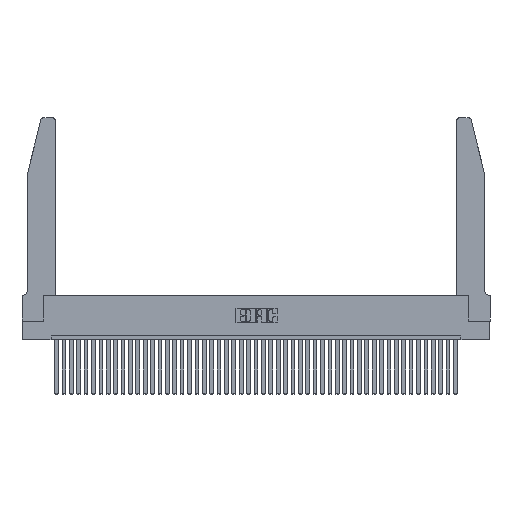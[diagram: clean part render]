
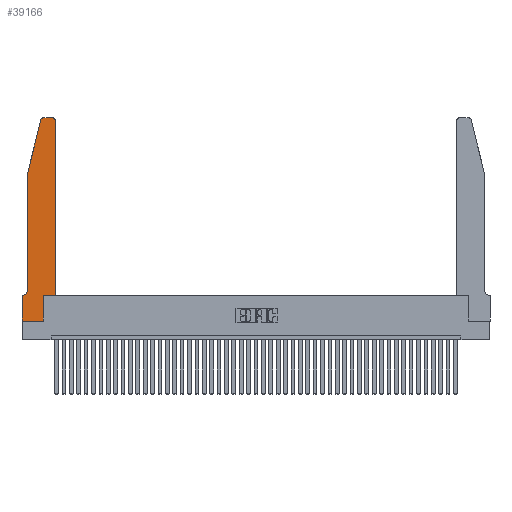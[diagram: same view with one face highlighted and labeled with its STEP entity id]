
A CAD part, top view. The second image highlights one B-rep face of the part: STEP entity #39166.
In plain terms, the highlighted planar face has unit normal (0, 0, 1).
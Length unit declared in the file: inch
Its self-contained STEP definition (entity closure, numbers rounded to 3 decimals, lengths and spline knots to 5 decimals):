
#9 = CARTESIAN_POINT ( 'NONE',  ( 0.0055, 0.42, 0.37 ) ) ;
#108 = CARTESIAN_POINT ( 'NONE',  ( 0.0755, 2., 0.37 ) ) ;
#1256 = CARTESIAN_POINT ( 'NONE',  ( 0.4205, 2.75, 0.37 ) ) ;
#1300 = DIRECTION ( 'NONE',  ( 1., 0., 0. ) ) ;
#1984 = VERTEX_POINT ( 'NONE', #10881 ) ;
#2824 = CARTESIAN_POINT ( 'NONE',  ( 0., 0.35, 0.37 ) ) ;
#2923 = LINE ( 'NONE', #6059, #33946 ) ;
#2985 = EDGE_CURVE ( 'NONE', #41878, #21738, #17395, .T. ) ;
#4377 = CARTESIAN_POINT ( 'NONE',  ( 0., 0.35, 0.37 ) ) ;
#4816 = CARTESIAN_POINT ( 'NONE',  ( 0.0755, 2., 0.37 ) ) ;
#5029 = VECTOR ( 'NONE', #18848, 39.37008 ) ;
#5049 = LINE ( 'NONE', #5074, #27039 ) ;
#5074 = CARTESIAN_POINT ( 'NONE',  ( 0.0755, 2., 0.37 ) ) ;
#5537 = VERTEX_POINT ( 'NONE', #5894 ) ;
#5815 = VERTEX_POINT ( 'NONE', #25529 ) ;
#5894 = CARTESIAN_POINT ( 'NONE',  ( 0., 0., 0.37 ) ) ;
#6059 = CARTESIAN_POINT ( 'NONE',  ( 0., 0., 0.37 ) ) ;
#7155 = VECTOR ( 'NONE', #27680, 39.37008 ) ;
#7263 = ORIENTED_EDGE ( 'NONE', *, *, #20639, .T. ) ;
#7273 = ORIENTED_EDGE ( 'NONE', *, *, #2985, .T. ) ;
#8125 = PLANE ( 'NONE',  #23287 ) ;
#8174 = DIRECTION ( 'NONE',  ( -1., 0., 0. ) ) ;
#9148 = ORIENTED_EDGE ( 'NONE', *, *, #26729, .T. ) ;
#9227 = DIRECTION ( 'NONE',  ( 0., -1., 0. ) ) ;
#9733 = EDGE_CURVE ( 'NONE', #5815, #37742, #29258, .T. ) ;
#10742 = CARTESIAN_POINT ( 'NONE',  ( 0.2605, 2.75, 0.37 ) ) ;
#10881 = CARTESIAN_POINT ( 'NONE',  ( 0.0755, 0.42, 0.37 ) ) ;
#10886 = EDGE_LOOP ( 'NONE', ( #37400, #36214, #31388, #26206, #20294, #7263, #9148, #14751, #7273, #43593, #41865, #40625 ) ) ;
#11112 = AXIS2_PLACEMENT_3D ( 'NONE', #23841, #27307, #30699 ) ;
#11327 = CARTESIAN_POINT ( 'NONE',  ( 0.4505, 0.35, 0.37 ) ) ;
#11474 = CARTESIAN_POINT ( 'NONE',  ( 0., 0., 0.37 ) ) ;
#13415 = EDGE_CURVE ( 'NONE', #23583, #5815, #24755, .T. ) ;
#13886 = LINE ( 'NONE', #4816, #30492 ) ;
#14198 = DIRECTION ( 'NONE',  ( 0., 0., -1. ) ) ;
#14213 = EDGE_CURVE ( 'NONE', #37742, #35950, #34302, .T. ) ;
#14751 = ORIENTED_EDGE ( 'NONE', *, *, #35418, .T. ) ;
#15029 = DIRECTION ( 'NONE',  ( 0., 0., 1. ) ) ;
#15263 = CARTESIAN_POINT ( 'NONE',  ( 0.4505, 0.35, 0.37 ) ) ;
#15727 = LINE ( 'NONE', #11474, #39719 ) ;
#17077 = DIRECTION ( 'NONE',  ( -1., 0., 0. ) ) ;
#17395 = LINE ( 'NONE', #36255, #5029 ) ;
#18848 = DIRECTION ( 'NONE',  ( 0., 1., 0. ) ) ;
#19045 = CIRCLE ( 'NONE', #31973, 0.07 ) ;
#19612 = DIRECTION ( 'NONE',  ( 1., 0., 0. ) ) ;
#19721 = CARTESIAN_POINT ( 'NONE',  ( 0.25487, 2.72718, 0.37 ) ) ;
#20294 = ORIENTED_EDGE ( 'NONE', *, *, #34423, .T. ) ;
#20495 = EDGE_CURVE ( 'NONE', #31347, #23967, #5049, .T. ) ;
#20639 = EDGE_CURVE ( 'NONE', #40526, #27176, #22181, .T. ) ;
#21601 = CARTESIAN_POINT ( 'NONE',  ( 0.2865, 0., 0.37 ) ) ;
#21650 = DIRECTION ( 'NONE',  ( 0., 1., 0. ) ) ;
#21738 = VERTEX_POINT ( 'NONE', #36974 ) ;
#22181 = LINE ( 'NONE', #30496, #7155 ) ;
#22701 = CARTESIAN_POINT ( 'NONE',  ( 0.0055, 0.35, 0.37 ) ) ;
#23287 = AXIS2_PLACEMENT_3D ( 'NONE', #4377, #15029, #38877 ) ;
#23583 = VERTEX_POINT ( 'NONE', #15263 ) ;
#23841 = CARTESIAN_POINT ( 'NONE',  ( 0.4205, 2.72, 0.37 ) ) ;
#23967 = VERTEX_POINT ( 'NONE', #108 ) ;
#24738 = CARTESIAN_POINT ( 'NONE',  ( 0.284, 2.75, 0.37 ) ) ;
#24755 = LINE ( 'NONE', #11327, #42322 ) ;
#24767 = VECTOR ( 'NONE', #42354, 39.37008 ) ;
#25082 = CARTESIAN_POINT ( 'NONE',  ( 0.4505, 0.35, 0.37 ) ) ;
#25529 = CARTESIAN_POINT ( 'NONE',  ( 0.4505, 2.72, 0.37 ) ) ;
#26206 = ORIENTED_EDGE ( 'NONE', *, *, #43778, .T. ) ;
#26729 = EDGE_CURVE ( 'NONE', #27176, #5537, #2923, .T. ) ;
#27039 = VECTOR ( 'NONE', #35727, 39.37008 ) ;
#27176 = VERTEX_POINT ( 'NONE', #2824 ) ;
#27307 = DIRECTION ( 'NONE',  ( 0., 0., 1. ) ) ;
#27680 = DIRECTION ( 'NONE',  ( -1., 0., 0. ) ) ;
#29258 = CIRCLE ( 'NONE', #11112, 0.03 ) ;
#30125 = LINE ( 'NONE', #25082, #24767 ) ;
#30492 = VECTOR ( 'NONE', #35772, 39.37008 ) ;
#30496 = CARTESIAN_POINT ( 'NONE',  ( 0.0755, 0.35, 0.37 ) ) ;
#30699 = DIRECTION ( 'NONE',  ( 1., 0., 0. ) ) ;
#30904 = EDGE_CURVE ( 'NONE', #35950, #31347, #38834, .T. ) ;
#31347 = VERTEX_POINT ( 'NONE', #19721 ) ;
#31388 = ORIENTED_EDGE ( 'NONE', *, *, #20495, .T. ) ;
#31973 = AXIS2_PLACEMENT_3D ( 'NONE', #9, #14198, #17077 ) ;
#33946 = VECTOR ( 'NONE', #9227, 39.37008 ) ;
#34302 = LINE ( 'NONE', #10742, #36940 ) ;
#34423 = EDGE_CURVE ( 'NONE', #1984, #40526, #19045, .T. ) ;
#34670 = FACE_OUTER_BOUND ( 'NONE', #10886, .T. ) ;
#35418 = EDGE_CURVE ( 'NONE', #5537, #41878, #15727, .T. ) ;
#35727 = DIRECTION ( 'NONE',  ( -0.239, -0.971, 0. ) ) ;
#35772 = DIRECTION ( 'NONE',  ( 0., -1., 0. ) ) ;
#35950 = VERTEX_POINT ( 'NONE', #24738 ) ;
#36214 = ORIENTED_EDGE ( 'NONE', *, *, #30904, .T. ) ;
#36255 = CARTESIAN_POINT ( 'NONE',  ( 0.2865, 0.35, 0.37 ) ) ;
#36940 = VECTOR ( 'NONE', #8174, 39.37008 ) ;
#36974 = CARTESIAN_POINT ( 'NONE',  ( 0.2865, 0.35, 0.37 ) ) ;
#37400 = ORIENTED_EDGE ( 'NONE', *, *, #14213, .T. ) ;
#37742 = VERTEX_POINT ( 'NONE', #1256 ) ;
#38834 = CIRCLE ( 'NONE', #40679, 0.03 ) ;
#38877 = DIRECTION ( 'NONE',  ( 1., 0., 0. ) ) ;
#39166 = ADVANCED_FACE ( 'NONE', ( #34670 ), #8125, .T. ) ;
#39713 = CARTESIAN_POINT ( 'NONE',  ( 0.284, 2.72, 0.37 ) ) ;
#39719 = VECTOR ( 'NONE', #1300, 39.37008 ) ;
#40526 = VERTEX_POINT ( 'NONE', #22701 ) ;
#40625 = ORIENTED_EDGE ( 'NONE', *, *, #9733, .T. ) ;
#40679 = AXIS2_PLACEMENT_3D ( 'NONE', #39713, #43152, #19612 ) ;
#41263 = EDGE_CURVE ( 'NONE', #21738, #23583, #30125, .T. ) ;
#41865 = ORIENTED_EDGE ( 'NONE', *, *, #13415, .T. ) ;
#41878 = VERTEX_POINT ( 'NONE', #21601 ) ;
#42322 = VECTOR ( 'NONE', #21650, 39.37008 ) ;
#42354 = DIRECTION ( 'NONE',  ( 1., 0., 0. ) ) ;
#43152 = DIRECTION ( 'NONE',  ( 0., 0., 1. ) ) ;
#43593 = ORIENTED_EDGE ( 'NONE', *, *, #41263, .T. ) ;
#43778 = EDGE_CURVE ( 'NONE', #23967, #1984, #13886, .T. ) ;
